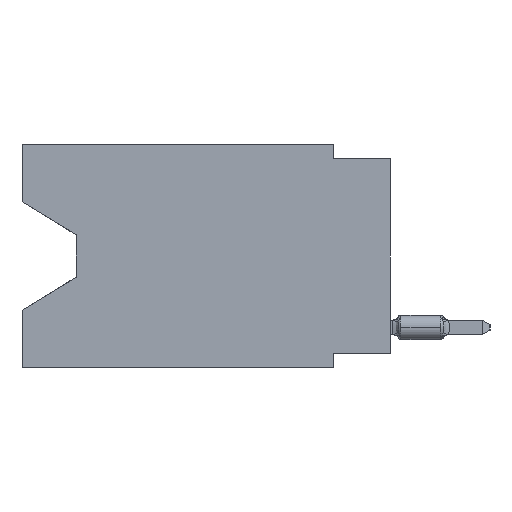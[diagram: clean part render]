
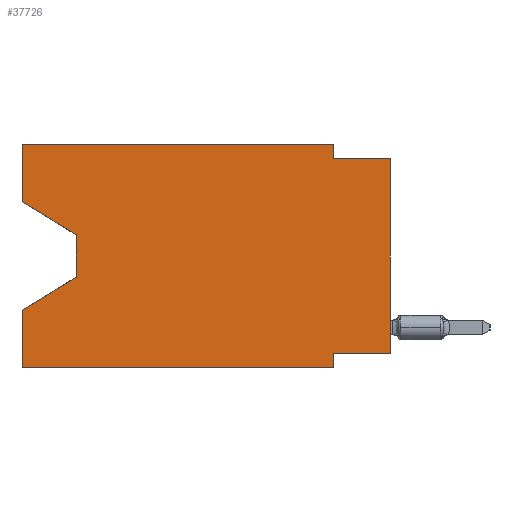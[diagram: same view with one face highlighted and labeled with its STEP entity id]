
A CAD part, left-side view. The second image highlights one B-rep face of the part: STEP entity #37726.
In plain terms, the highlighted planar face has unit normal (-1, 0, 0).
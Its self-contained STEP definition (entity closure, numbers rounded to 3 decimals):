
#2404 = CARTESIAN_POINT ( 'NONE',  ( 0., 16.383, -2.546 ) ) ;
#2684 = VECTOR ( 'NONE', #15250, 1000. ) ;
#3999 = EDGE_CURVE ( 'NONE', #18250, #12182, #78510, .T. ) ;
#4626 = LINE ( 'NONE', #74834, #28877 ) ;
#5698 = CARTESIAN_POINT ( 'NONE',  ( 0., 2.54, -0.635 ) ) ;
#9625 = EDGE_CURVE ( 'NONE', #79361, #11552, #35554, .T. ) ;
#10597 = EDGE_CURVE ( 'NONE', #79361, #58267, #13084, .T. ) ;
#11218 = CARTESIAN_POINT ( 'NONE',  ( 0., 16.383, -7.36 ) ) ;
#11552 = VERTEX_POINT ( 'NONE', #75022 ) ;
#12182 = VERTEX_POINT ( 'NONE', #42111 ) ;
#12426 = ORIENTED_EDGE ( 'NONE', *, *, #61349, .F. ) ;
#12559 = DIRECTION ( 'NONE',  ( 0., 0., -1. ) ) ;
#12583 = DIRECTION ( 'NONE',  ( 0., 0., -1. ) ) ;
#12819 = ORIENTED_EDGE ( 'NONE', *, *, #16071, .F. ) ;
#13084 = LINE ( 'NONE', #64068, #21571 ) ;
#13315 = VECTOR ( 'NONE', #12583, 1000. ) ;
#13688 = ORIENTED_EDGE ( 'NONE', *, *, #54628, .F. ) ;
#14584 = CARTESIAN_POINT ( 'NONE',  ( 0., 0., 0. ) ) ;
#15250 = DIRECTION ( 'NONE',  ( 0., -1., 0. ) ) ;
#16071 = EDGE_CURVE ( 'NONE', #51129, #12182, #69174, .T. ) ;
#18250 = VERTEX_POINT ( 'NONE', #65599 ) ;
#19654 = DIRECTION ( 'NONE',  ( 0., 0.855, -0.519 ) ) ;
#19960 = AXIS2_PLACEMENT_3D ( 'NONE', #30615, #54551, #22786 ) ;
#19987 = ORIENTED_EDGE ( 'NONE', *, *, #63792, .F. ) ;
#20140 = LINE ( 'NONE', #76576, #38869 ) ;
#21571 = VECTOR ( 'NONE', #71155, 1000. ) ;
#22048 = ORIENTED_EDGE ( 'NONE', *, *, #77744, .T. ) ;
#22195 = ORIENTED_EDGE ( 'NONE', *, *, #24105, .F. ) ;
#22786 = DIRECTION ( 'NONE',  ( 0., 0., -1. ) ) ;
#24105 = EDGE_CURVE ( 'NONE', #18250, #44933, #25785, .T. ) ;
#24322 = ORIENTED_EDGE ( 'NONE', *, *, #72218, .T. ) ;
#24347 = FACE_OUTER_BOUND ( 'NONE', #42876, .T. ) ;
#25188 = CARTESIAN_POINT ( 'NONE',  ( 0., 2.54, -9.906 ) ) ;
#25785 = LINE ( 'NONE', #51263, #36656 ) ;
#25906 = ORIENTED_EDGE ( 'NONE', *, *, #9625, .F. ) ;
#28877 = VECTOR ( 'NONE', #12559, 1000. ) ;
#29249 = VERTEX_POINT ( 'NONE', #25188 ) ;
#29367 = ORIENTED_EDGE ( 'NONE', *, *, #10597, .T. ) ;
#29585 = ORIENTED_EDGE ( 'NONE', *, *, #66167, .T. ) ;
#29909 = CARTESIAN_POINT ( 'NONE',  ( 0., 13.97, -4.013 ) ) ;
#30121 = CARTESIAN_POINT ( 'NONE',  ( 0., 16.383, 0. ) ) ;
#30615 = CARTESIAN_POINT ( 'NONE',  ( 0., 16.383, 0. ) ) ;
#30814 = VECTOR ( 'NONE', #41818, 1000. ) ;
#35554 = LINE ( 'NONE', #30121, #30814 ) ;
#36544 = LINE ( 'NONE', #75398, #65856 ) ;
#36656 = VECTOR ( 'NONE', #82194, 1000. ) ;
#36873 = VECTOR ( 'NONE', #41289, 1000. ) ;
#37130 = VECTOR ( 'NONE', #49950, 1000. ) ;
#37294 = PLANE ( 'NONE',  #19960 ) ;
#37726 = ADVANCED_FACE ( 'NONE', ( #24347 ), #37294, .F. ) ;
#38061 = LINE ( 'NONE', #75685, #13315 ) ;
#38869 = VECTOR ( 'NONE', #57777, 1000. ) ;
#40731 = LINE ( 'NONE', #59985, #2684 ) ;
#41289 = DIRECTION ( 'NONE',  ( 0., 0., 1. ) ) ;
#41818 = DIRECTION ( 'NONE',  ( 0., 0., 1. ) ) ;
#42111 = CARTESIAN_POINT ( 'NONE',  ( 0., 0., -0.635 ) ) ;
#42876 = EDGE_LOOP ( 'NONE', ( #29367, #29585, #22048, #12426, #24322, #63684, #22195, #62091, #12819, #19987, #13688, #25906 ) ) ;
#43724 = CARTESIAN_POINT ( 'NONE',  ( 0., 2.54, 0. ) ) ;
#44933 = VERTEX_POINT ( 'NONE', #60415 ) ;
#46371 = LINE ( 'NONE', #76897, #77842 ) ;
#47843 = VECTOR ( 'NONE', #78650, 1000. ) ;
#49078 = DIRECTION ( 'NONE',  ( 0., 0., -1. ) ) ;
#49252 = CARTESIAN_POINT ( 'NONE',  ( 0., 16.383, 0. ) ) ;
#49950 = DIRECTION ( 'NONE',  ( 0., -1., 0. ) ) ;
#51129 = VERTEX_POINT ( 'NONE', #5698 ) ;
#51263 = CARTESIAN_POINT ( 'NONE',  ( 0., 0., -9.271 ) ) ;
#54551 = DIRECTION ( 'NONE',  ( 1., 0., 0. ) ) ;
#54568 = CARTESIAN_POINT ( 'NONE',  ( 0., 0., -0.635 ) ) ;
#54628 = EDGE_CURVE ( 'NONE', #11552, #79721, #74324, .T. ) ;
#56728 = VERTEX_POINT ( 'NONE', #69960 ) ;
#57777 = DIRECTION ( 'NONE',  ( 0., 0., 1. ) ) ;
#58267 = VERTEX_POINT ( 'NONE', #29909 ) ;
#59985 = CARTESIAN_POINT ( 'NONE',  ( 0., 16.383, -9.906 ) ) ;
#60415 = CARTESIAN_POINT ( 'NONE',  ( 0., 2.54, -9.271 ) ) ;
#61349 = EDGE_CURVE ( 'NONE', #56728, #81683, #20140, .T. ) ;
#62091 = ORIENTED_EDGE ( 'NONE', *, *, #3999, .T. ) ;
#63684 = ORIENTED_EDGE ( 'NONE', *, *, #71622, .F. ) ;
#63792 = EDGE_CURVE ( 'NONE', #79721, #51129, #36544, .T. ) ;
#64068 = CARTESIAN_POINT ( 'NONE',  ( 0., 16.383, -2.546 ) ) ;
#65599 = CARTESIAN_POINT ( 'NONE',  ( 0., 0., -9.271 ) ) ;
#65856 = VECTOR ( 'NONE', #49078, 1000. ) ;
#66167 = EDGE_CURVE ( 'NONE', #58267, #76942, #4626, .T. ) ;
#66795 = CARTESIAN_POINT ( 'NONE',  ( 0., 13.97, -5.893 ) ) ;
#69174 = LINE ( 'NONE', #54568, #37130 ) ;
#69960 = CARTESIAN_POINT ( 'NONE',  ( 0., 16.383, -9.906 ) ) ;
#71155 = DIRECTION ( 'NONE',  ( 0., -0.855, -0.519 ) ) ;
#71622 = EDGE_CURVE ( 'NONE', #44933, #29249, #38061, .T. ) ;
#72218 = EDGE_CURVE ( 'NONE', #56728, #29249, #40731, .T. ) ;
#74324 = LINE ( 'NONE', #49252, #47843 ) ;
#74834 = CARTESIAN_POINT ( 'NONE',  ( 0., 13.97, -4.013 ) ) ;
#75022 = CARTESIAN_POINT ( 'NONE',  ( 0., 16.383, 0. ) ) ;
#75398 = CARTESIAN_POINT ( 'NONE',  ( 0., 2.54, 0. ) ) ;
#75685 = CARTESIAN_POINT ( 'NONE',  ( 0., 2.54, -9.906 ) ) ;
#76576 = CARTESIAN_POINT ( 'NONE',  ( 0., 16.383, 0. ) ) ;
#76897 = CARTESIAN_POINT ( 'NONE',  ( 0., 13.97, -5.893 ) ) ;
#76942 = VERTEX_POINT ( 'NONE', #66795 ) ;
#77744 = EDGE_CURVE ( 'NONE', #76942, #81683, #46371, .T. ) ;
#77842 = VECTOR ( 'NONE', #19654, 1000. ) ;
#78510 = LINE ( 'NONE', #14584, #36873 ) ;
#78650 = DIRECTION ( 'NONE',  ( 0., -1., 0. ) ) ;
#79361 = VERTEX_POINT ( 'NONE', #2404 ) ;
#79721 = VERTEX_POINT ( 'NONE', #43724 ) ;
#81683 = VERTEX_POINT ( 'NONE', #11218 ) ;
#82194 = DIRECTION ( 'NONE',  ( 0., 1., 0. ) ) ;
